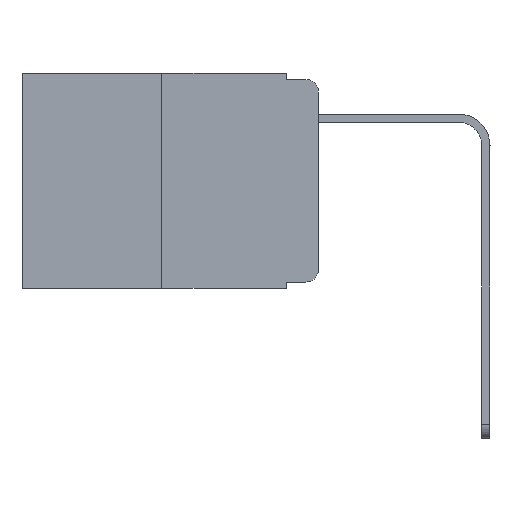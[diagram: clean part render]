
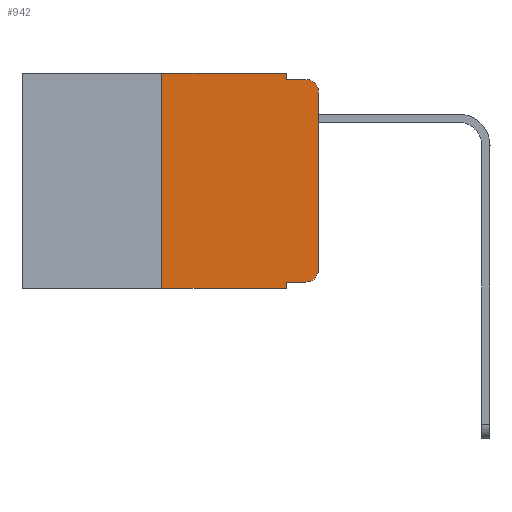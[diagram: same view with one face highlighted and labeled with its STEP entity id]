
A CAD part, left-side view. The second image highlights one B-rep face of the part: STEP entity #942.
In plain terms, the highlighted planar face has unit normal (-1, 0, 0).
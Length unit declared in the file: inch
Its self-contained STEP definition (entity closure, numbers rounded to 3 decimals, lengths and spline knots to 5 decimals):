
#279 = LINE ( 'NONE', #21809, #21881 ) ;
#330 = CARTESIAN_POINT ( 'NONE',  ( 0., 0.473, -0.343 ) ) ;
#502 = VERTEX_POINT ( 'NONE', #10022 ) ;
#838 = LINE ( 'NONE', #874, #4738 ) ;
#874 = CARTESIAN_POINT ( 'NONE',  ( 0., 0.051, -0.333 ) ) ;
#942 = ADVANCED_FACE ( 'NONE', ( #9641 ), #17235, .F. ) ;
#1078 = CARTESIAN_POINT ( 'NONE',  ( 0., 0.473, 0. ) ) ;
#1312 = DIRECTION ( 'NONE',  ( 0., 0., -1. ) ) ;
#2097 = DIRECTION ( 'NONE',  ( 0., -1., 0. ) ) ;
#2160 = VERTEX_POINT ( 'NONE', #16965 ) ;
#2176 = LINE ( 'NONE', #12308, #2461 ) ;
#2461 = VECTOR ( 'NONE', #6515, 39.37008 ) ;
#2528 = DIRECTION ( 'NONE',  ( 0., 0., -1. ) ) ;
#2568 = CIRCLE ( 'NONE', #3393, 0.02 ) ;
#3068 = EDGE_LOOP ( 'NONE', ( #17150, #5620, #10143, #15439, #13238, #12942, #17210, #15794, #5129, #15686 ) ) ;
#3143 = DIRECTION ( 'NONE',  ( 1., 0., 0. ) ) ;
#3393 = AXIS2_PLACEMENT_3D ( 'NONE', #8360, #17576, #6087 ) ;
#3796 = VERTEX_POINT ( 'NONE', #7280 ) ;
#3956 = VERTEX_POINT ( 'NONE', #9422 ) ;
#4286 = LINE ( 'NONE', #15764, #21987 ) ;
#4550 = CARTESIAN_POINT ( 'NONE',  ( 0., 0.051, 0. ) ) ;
#4637 = DIRECTION ( 'NONE',  ( 0., 0., -1. ) ) ;
#4738 = VECTOR ( 'NONE', #10356, 39.37008 ) ;
#5112 = EDGE_CURVE ( 'NONE', #11406, #5792, #19358, .T. ) ;
#5129 = ORIENTED_EDGE ( 'NONE', *, *, #15914, .T. ) ;
#5140 = EDGE_CURVE ( 'NONE', #22015, #3956, #21448, .T. ) ;
#5620 = ORIENTED_EDGE ( 'NONE', *, *, #5140, .T. ) ;
#5792 = VERTEX_POINT ( 'NONE', #10837 ) ;
#6087 = DIRECTION ( 'NONE',  ( 0., 0., -1. ) ) ;
#6319 = DIRECTION ( 'NONE',  ( -1., 0., 0. ) ) ;
#6515 = DIRECTION ( 'NONE',  ( 0., 0., 1. ) ) ;
#7142 = VECTOR ( 'NONE', #10448, 39.37008 ) ;
#7280 = CARTESIAN_POINT ( 'NONE',  ( 0., 0., -0.313 ) ) ;
#7362 = CARTESIAN_POINT ( 'NONE',  ( 0., 0.25, 0. ) ) ;
#7682 = CARTESIAN_POINT ( 'NONE',  ( 0., 0.051, -0.333 ) ) ;
#8086 = CARTESIAN_POINT ( 'NONE',  ( 0., 0.25, -0.343 ) ) ;
#8360 = CARTESIAN_POINT ( 'NONE',  ( 0., 0.02, -0.313 ) ) ;
#8513 = CARTESIAN_POINT ( 'NONE',  ( 0., 0.02, -0.03 ) ) ;
#8695 = EDGE_CURVE ( 'NONE', #3796, #22015, #279, .T. ) ;
#9422 = CARTESIAN_POINT ( 'NONE',  ( 0., 0.02, -0.01 ) ) ;
#9576 = VECTOR ( 'NONE', #2097, 39.37008 ) ;
#9641 = FACE_OUTER_BOUND ( 'NONE', #3068, .T. ) ;
#10022 = CARTESIAN_POINT ( 'NONE',  ( 0., 0.051, -0.343 ) ) ;
#10143 = ORIENTED_EDGE ( 'NONE', *, *, #18442, .F. ) ;
#10356 = DIRECTION ( 'NONE',  ( 0., -1., 0. ) ) ;
#10448 = DIRECTION ( 'NONE',  ( 0., 0., -1. ) ) ;
#10837 = CARTESIAN_POINT ( 'NONE',  ( 0., 0.051, -0.01 ) ) ;
#11406 = VERTEX_POINT ( 'NONE', #22754 ) ;
#11825 = AXIS2_PLACEMENT_3D ( 'NONE', #8513, #6319, #4637 ) ;
#12308 = CARTESIAN_POINT ( 'NONE',  ( 0., 0.25, 0. ) ) ;
#12723 = CARTESIAN_POINT ( 'NONE',  ( 0., 0.473, 0. ) ) ;
#12942 = ORIENTED_EDGE ( 'NONE', *, *, #13007, .F. ) ;
#13007 = EDGE_CURVE ( 'NONE', #13503, #17528, #2176, .T. ) ;
#13114 = LINE ( 'NONE', #14142, #7142 ) ;
#13238 = ORIENTED_EDGE ( 'NONE', *, *, #17339, .F. ) ;
#13427 = VERTEX_POINT ( 'NONE', #7682 ) ;
#13503 = VERTEX_POINT ( 'NONE', #8086 ) ;
#14142 = CARTESIAN_POINT ( 'NONE',  ( 0., 0.051, 0. ) ) ;
#14293 = VECTOR ( 'NONE', #2528, 39.37008 ) ;
#14689 = LINE ( 'NONE', #330, #9576 ) ;
#15144 = EDGE_CURVE ( 'NONE', #13503, #502, #14689, .T. ) ;
#15439 = ORIENTED_EDGE ( 'NONE', *, *, #5112, .F. ) ;
#15650 = CARTESIAN_POINT ( 'NONE',  ( 0., 0., -0.03 ) ) ;
#15686 = ORIENTED_EDGE ( 'NONE', *, *, #24611, .T. ) ;
#15764 = CARTESIAN_POINT ( 'NONE',  ( 0., 0.051, -0.01 ) ) ;
#15794 = ORIENTED_EDGE ( 'NONE', *, *, #16040, .F. ) ;
#15914 = EDGE_CURVE ( 'NONE', #13427, #2160, #838, .T. ) ;
#16040 = EDGE_CURVE ( 'NONE', #13427, #502, #13114, .T. ) ;
#16236 = DIRECTION ( 'NONE',  ( 0., -1., 0. ) ) ;
#16965 = CARTESIAN_POINT ( 'NONE',  ( 0., 0.02, -0.333 ) ) ;
#17150 = ORIENTED_EDGE ( 'NONE', *, *, #8695, .T. ) ;
#17210 = ORIENTED_EDGE ( 'NONE', *, *, #15144, .T. ) ;
#17235 = PLANE ( 'NONE',  #21996 ) ;
#17339 = EDGE_CURVE ( 'NONE', #17528, #11406, #18765, .T. ) ;
#17528 = VERTEX_POINT ( 'NONE', #7362 ) ;
#17576 = DIRECTION ( 'NONE',  ( -1., 0., 0. ) ) ;
#18442 = EDGE_CURVE ( 'NONE', #5792, #3956, #4286, .T. ) ;
#18459 = DIRECTION ( 'NONE',  ( 0., 0., 1. ) ) ;
#18765 = LINE ( 'NONE', #1078, #24716 ) ;
#19358 = LINE ( 'NONE', #4550, #14293 ) ;
#19531 = DIRECTION ( 'NONE',  ( 0., -1., 0. ) ) ;
#21448 = CIRCLE ( 'NONE', #11825, 0.02 ) ;
#21809 = CARTESIAN_POINT ( 'NONE',  ( 0., 0., 0. ) ) ;
#21881 = VECTOR ( 'NONE', #18459, 39.37008 ) ;
#21987 = VECTOR ( 'NONE', #19531, 39.37008 ) ;
#21996 = AXIS2_PLACEMENT_3D ( 'NONE', #12723, #3143, #1312 ) ;
#22015 = VERTEX_POINT ( 'NONE', #15650 ) ;
#22754 = CARTESIAN_POINT ( 'NONE',  ( 0., 0.051, 0. ) ) ;
#24611 = EDGE_CURVE ( 'NONE', #2160, #3796, #2568, .T. ) ;
#24716 = VECTOR ( 'NONE', #16236, 39.37008 ) ;
